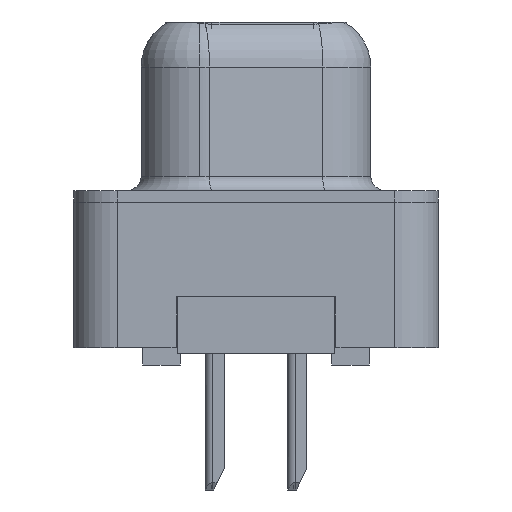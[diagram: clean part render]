
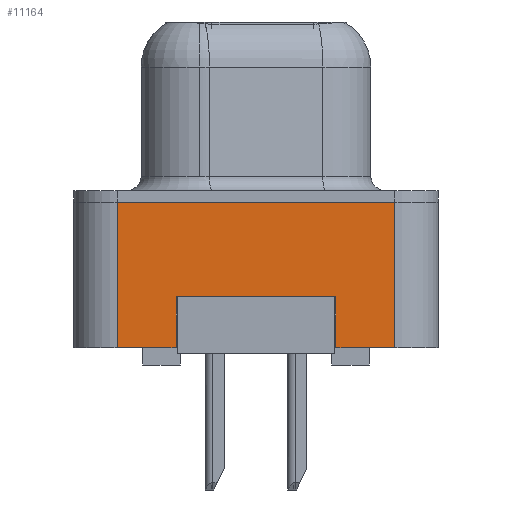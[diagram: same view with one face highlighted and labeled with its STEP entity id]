
A CAD part, left-side view. The second image highlights one B-rep face of the part: STEP entity #11164.
In plain terms, the highlighted planar face has unit normal (-1, 0, 0).
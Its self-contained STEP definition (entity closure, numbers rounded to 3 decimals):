
#307 = DIRECTION ( 'NONE',  ( 0., -1., 0. ) ) ;
#1126 = VERTEX_POINT ( 'NONE', #11868 ) ;
#2140 = EDGE_CURVE ( 'NONE', #1126, #2982, #6902, .T. ) ;
#2172 = CARTESIAN_POINT ( 'NONE',  ( -2.995, -4.775, -5. ) ) ;
#2285 = ORIENTED_EDGE ( 'NONE', *, *, #15524, .F. ) ;
#2415 = CARTESIAN_POINT ( 'NONE',  ( -2.995, 4.775, 0. ) ) ;
#2626 = ORIENTED_EDGE ( 'NONE', *, *, #12525, .T. ) ;
#2982 = VERTEX_POINT ( 'NONE', #14993 ) ;
#3070 = DIRECTION ( 'NONE',  ( 0., 0., 1. ) ) ;
#3239 = CARTESIAN_POINT ( 'NONE',  ( -2.995, -2.75, -3.25 ) ) ;
#3332 = VECTOR ( 'NONE', #6971, 1000. ) ;
#4893 = LINE ( 'NONE', #3239, #14357 ) ;
#5141 = LINE ( 'NONE', #8582, #10545 ) ;
#5630 = AXIS2_PLACEMENT_3D ( 'NONE', #15808, #12558, #3070 ) ;
#5718 = LINE ( 'NONE', #5822, #3332 ) ;
#5822 = CARTESIAN_POINT ( 'NONE',  ( -2.995, 4.775, -5. ) ) ;
#6092 = EDGE_CURVE ( 'NONE', #20418, #2982, #5141, .T. ) ;
#6472 = PLANE ( 'NONE',  #5630 ) ;
#6633 = DIRECTION ( 'NONE',  ( 0., 0., 1. ) ) ;
#6902 = LINE ( 'NONE', #13295, #17458 ) ;
#6971 = DIRECTION ( 'NONE',  ( 0., 0., 1. ) ) ;
#7290 = LINE ( 'NONE', #17136, #17603 ) ;
#7453 = CARTESIAN_POINT ( 'NONE',  ( -2.995, 2.75, -3.25 ) ) ;
#8057 = VERTEX_POINT ( 'NONE', #16091 ) ;
#8475 = VERTEX_POINT ( 'NONE', #17526 ) ;
#8582 = CARTESIAN_POINT ( 'NONE',  ( -2.995, 2.75, -3.25 ) ) ;
#8688 = VECTOR ( 'NONE', #307, 1000. ) ;
#8953 = VECTOR ( 'NONE', #6633, 1000. ) ;
#9104 = VERTEX_POINT ( 'NONE', #10900 ) ;
#9673 = LINE ( 'NONE', #2172, #8688 ) ;
#9869 = LINE ( 'NONE', #11247, #8953 ) ;
#9993 = EDGE_CURVE ( 'NONE', #8057, #20418, #10183, .T. ) ;
#10183 = LINE ( 'NONE', #13234, #10942 ) ;
#10442 = VERTEX_POINT ( 'NONE', #18121 ) ;
#10545 = VECTOR ( 'NONE', #14775, 1000. ) ;
#10900 = CARTESIAN_POINT ( 'NONE',  ( -2.995, -4.775, 0. ) ) ;
#10942 = VECTOR ( 'NONE', #19706, 1000. ) ;
#11164 = ADVANCED_FACE ( 'NONE', ( #12461 ), #6472, .T. ) ;
#11247 = CARTESIAN_POINT ( 'NONE',  ( -2.995, -4.775, -5. ) ) ;
#11263 = DIRECTION ( 'NONE',  ( 0., 0., -1. ) ) ;
#11276 = ORIENTED_EDGE ( 'NONE', *, *, #13116, .T. ) ;
#11402 = DIRECTION ( 'NONE',  ( 0., -1., 0. ) ) ;
#11868 = CARTESIAN_POINT ( 'NONE',  ( -2.995, 4.775, -5. ) ) ;
#12061 = EDGE_CURVE ( 'NONE', #1126, #19219, #5718, .T. ) ;
#12461 = FACE_OUTER_BOUND ( 'NONE', #18327, .T. ) ;
#12525 = EDGE_CURVE ( 'NONE', #8057, #10442, #4893, .T. ) ;
#12558 = DIRECTION ( 'NONE',  ( -1., 0., 0. ) ) ;
#13116 = EDGE_CURVE ( 'NONE', #10442, #8475, #9673, .T. ) ;
#13234 = CARTESIAN_POINT ( 'NONE',  ( -2.995, 2.75, -3.25 ) ) ;
#13295 = CARTESIAN_POINT ( 'NONE',  ( -2.995, -4.775, -5. ) ) ;
#13299 = ORIENTED_EDGE ( 'NONE', *, *, #16831, .T. ) ;
#13942 = ORIENTED_EDGE ( 'NONE', *, *, #12061, .F. ) ;
#14357 = VECTOR ( 'NONE', #11263, 1000. ) ;
#14775 = DIRECTION ( 'NONE',  ( 0., 0., -1. ) ) ;
#14993 = CARTESIAN_POINT ( 'NONE',  ( -2.995, 2.75, -5. ) ) ;
#15524 = EDGE_CURVE ( 'NONE', #19219, #9104, #7290, .T. ) ;
#15808 = CARTESIAN_POINT ( 'NONE',  ( -2.995, -4.775, -5. ) ) ;
#16091 = CARTESIAN_POINT ( 'NONE',  ( -2.995, -2.75, -3.25 ) ) ;
#16831 = EDGE_CURVE ( 'NONE', #8475, #9104, #9869, .T. ) ;
#16926 = DIRECTION ( 'NONE',  ( 0., -1., 0. ) ) ;
#17136 = CARTESIAN_POINT ( 'NONE',  ( -2.995, -4.775, 0. ) ) ;
#17458 = VECTOR ( 'NONE', #11402, 1000. ) ;
#17526 = CARTESIAN_POINT ( 'NONE',  ( -2.995, -4.775, -5. ) ) ;
#17603 = VECTOR ( 'NONE', #16926, 1000. ) ;
#18121 = CARTESIAN_POINT ( 'NONE',  ( -2.995, -2.75, -5. ) ) ;
#18327 = EDGE_LOOP ( 'NONE', ( #2626, #11276, #13299, #2285, #13942, #18922, #20542, #20275 ) ) ;
#18922 = ORIENTED_EDGE ( 'NONE', *, *, #2140, .T. ) ;
#19219 = VERTEX_POINT ( 'NONE', #2415 ) ;
#19706 = DIRECTION ( 'NONE',  ( 0., 1., 0. ) ) ;
#20275 = ORIENTED_EDGE ( 'NONE', *, *, #9993, .F. ) ;
#20418 = VERTEX_POINT ( 'NONE', #7453 ) ;
#20542 = ORIENTED_EDGE ( 'NONE', *, *, #6092, .F. ) ;
